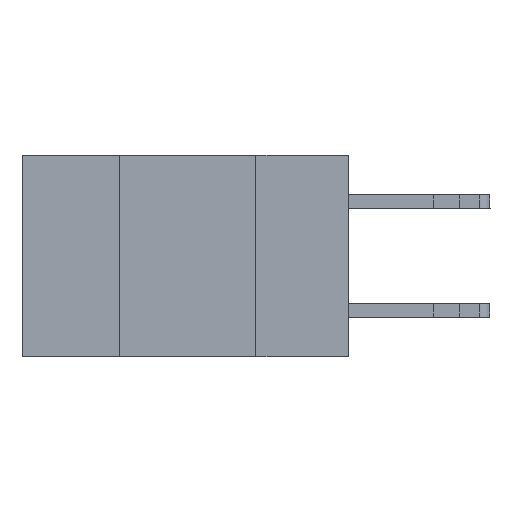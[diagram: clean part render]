
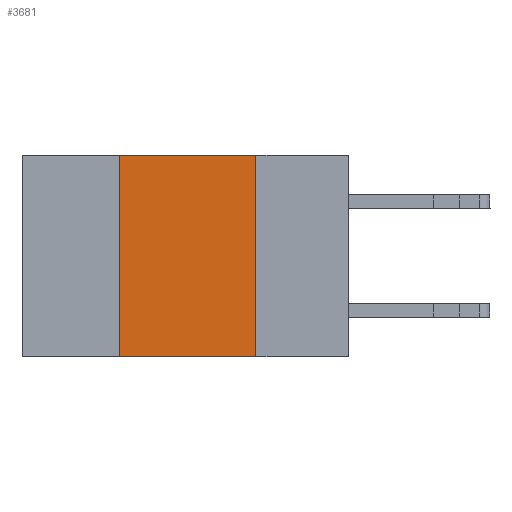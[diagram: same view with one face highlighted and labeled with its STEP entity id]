
A CAD part, left-side view. The second image highlights one B-rep face of the part: STEP entity #3681.
In plain terms, the highlighted planar face has unit normal (-1, 0, 0).
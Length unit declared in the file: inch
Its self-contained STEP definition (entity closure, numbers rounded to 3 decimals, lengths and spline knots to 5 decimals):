
#282 = ORIENTED_EDGE ( 'NONE', *, *, #11172, .F. ) ;
#424 = LINE ( 'NONE', #9093, #19333 ) ;
#486 = ORIENTED_EDGE ( 'NONE', *, *, #18184, .T. ) ;
#515 = LINE ( 'NONE', #2895, #18881 ) ;
#2469 = VECTOR ( 'NONE', #6109, 39.37008 ) ;
#2475 = CARTESIAN_POINT ( 'NONE',  ( 0., 0.17, -0.37 ) ) ;
#2895 = CARTESIAN_POINT ( 'NONE',  ( 0., 0.6, -0.37 ) ) ;
#3681 = ADVANCED_FACE ( 'NONE', ( #6646 ), #12880, .F. ) ;
#3937 = DIRECTION ( 'NONE',  ( 1., 0., 0. ) ) ;
#4374 = EDGE_CURVE ( 'NONE', #16853, #6743, #6322, .T. ) ;
#5582 = DIRECTION ( 'NONE',  ( 0., 0., 1. ) ) ;
#6109 = DIRECTION ( 'NONE',  ( 0., -1., 0. ) ) ;
#6232 = CARTESIAN_POINT ( 'NONE',  ( 0., 0.42, 0. ) ) ;
#6322 = LINE ( 'NONE', #2475, #19822 ) ;
#6501 = EDGE_LOOP ( 'NONE', ( #22065, #22111, #282, #486 ) ) ;
#6527 = VERTEX_POINT ( 'NONE', #16175 ) ;
#6646 = FACE_OUTER_BOUND ( 'NONE', #6501, .T. ) ;
#6743 = VERTEX_POINT ( 'NONE', #18592 ) ;
#7973 = VERTEX_POINT ( 'NONE', #6232 ) ;
#9093 = CARTESIAN_POINT ( 'NONE',  ( 0., 0.42, -0.37 ) ) ;
#9952 = EDGE_CURVE ( 'NONE', #7973, #16853, #20799, .T. ) ;
#11172 = EDGE_CURVE ( 'NONE', #6527, #7973, #424, .T. ) ;
#12880 = PLANE ( 'NONE',  #16813 ) ;
#13234 = DIRECTION ( 'NONE',  ( 0., 0., -1. ) ) ;
#14624 = CARTESIAN_POINT ( 'NONE',  ( 0., 0.6, 0. ) ) ;
#15170 = CARTESIAN_POINT ( 'NONE',  ( 0., 0.17, 0. ) ) ;
#16175 = CARTESIAN_POINT ( 'NONE',  ( 0., 0.42, -0.37 ) ) ;
#16357 = DIRECTION ( 'NONE',  ( 0., 0., -1. ) ) ;
#16813 = AXIS2_PLACEMENT_3D ( 'NONE', #14624, #3937, #16357 ) ;
#16853 = VERTEX_POINT ( 'NONE', #15170 ) ;
#18184 = EDGE_CURVE ( 'NONE', #6527, #6743, #515, .T. ) ;
#18413 = CARTESIAN_POINT ( 'NONE',  ( 0., 0.6, 0. ) ) ;
#18592 = CARTESIAN_POINT ( 'NONE',  ( 0., 0.17, -0.37 ) ) ;
#18881 = VECTOR ( 'NONE', #20650, 39.37008 ) ;
#19333 = VECTOR ( 'NONE', #5582, 39.37008 ) ;
#19822 = VECTOR ( 'NONE', #13234, 39.37008 ) ;
#20650 = DIRECTION ( 'NONE',  ( 0., -1., 0. ) ) ;
#20799 = LINE ( 'NONE', #18413, #2469 ) ;
#22065 = ORIENTED_EDGE ( 'NONE', *, *, #4374, .F. ) ;
#22111 = ORIENTED_EDGE ( 'NONE', *, *, #9952, .F. ) ;
